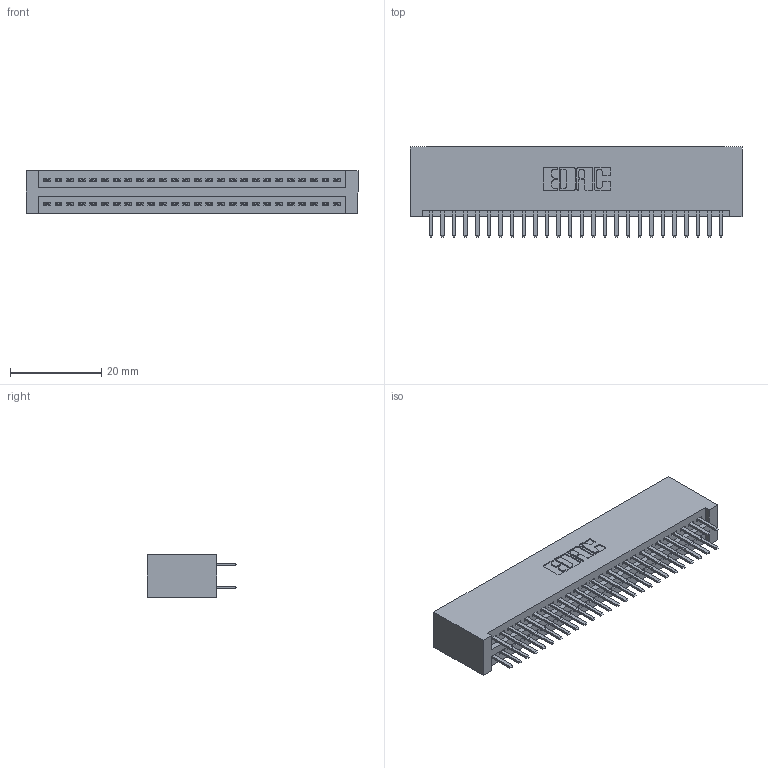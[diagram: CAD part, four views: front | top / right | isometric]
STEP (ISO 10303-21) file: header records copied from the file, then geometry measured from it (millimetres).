
FILE_DESCRIPTION (( 'STEP AP203' ), '1' );
FILE_NAME ('345-052-520-201.STEP', '2019-10-29T13:50:06', ( '' ), ( '' ), 'SwSTEP 2.0', 'SolidWorks 2016', '' );
FILE_SCHEMA (( 'CONFIG_CONTROL_DESIGN' ));
Length unit declared in the file: inch
Products named in the file (3): 345-052-520-201; 345 Part_No Mounting Lugs; 345-292-001_345-293-120
Assembly tree (53 placements, depth 2):
  345-052-520-201
    345 Part_No Mounting Lugs
    345-292-001_345-293-120  x52
Bounding box: 72.64 x 19.68 x 9.4 mm (x, y, z)
Volume: 7501.2 mm3; surface area: 11032.9 mm2
Topology: 53 solids, 53 shells, 2926 faces, 8481 edges, 5514 vertices
Faces by surface type: plane 1896, cylinder 1030
Entity records: 22391 total; most frequent: CARTESIAN_POINT 3780, ORIENTED_EDGE 3702, DIRECTION 3335, EDGE_CURVE 1851, LINE 1619, VECTOR 1619, VERTEX_POINT 1230, AXIS2_PLACEMENT_3D 858
